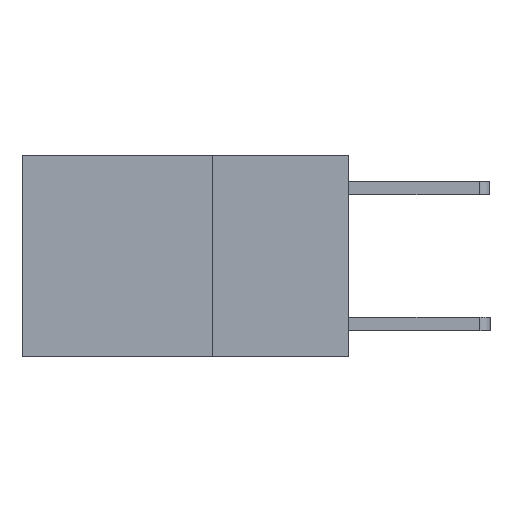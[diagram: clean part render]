
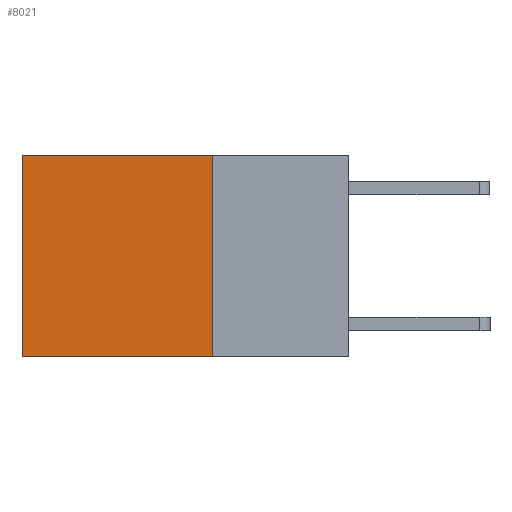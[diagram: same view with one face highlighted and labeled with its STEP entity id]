
A CAD part, left-side view. The second image highlights one B-rep face of the part: STEP entity #8021.
In plain terms, the highlighted planar face has unit normal (-1, 0, 0).
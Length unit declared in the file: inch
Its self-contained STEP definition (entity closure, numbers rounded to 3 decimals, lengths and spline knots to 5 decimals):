
#5 = VECTOR ( 'NONE', #6315, 39.37008 ) ;
#117 = LINE ( 'NONE', #4311, #6963 ) ;
#563 = EDGE_LOOP ( 'NONE', ( #4893, #7709, #1870, #7414 ) ) ;
#976 = CARTESIAN_POINT ( 'NONE',  ( 0.2625, 0.6, 0. ) ) ;
#1108 = LINE ( 'NONE', #2004, #7774 ) ;
#1376 = CARTESIAN_POINT ( 'NONE',  ( 0.2625, 0.25, 0. ) ) ;
#1395 = VECTOR ( 'NONE', #7328, 39.37008 ) ;
#1697 = LINE ( 'NONE', #1863, #5 ) ;
#1863 = CARTESIAN_POINT ( 'NONE',  ( 0.2625, 0.25, -0.37 ) ) ;
#1870 = ORIENTED_EDGE ( 'NONE', *, *, #1940, .F. ) ;
#1940 = EDGE_CURVE ( 'NONE', #6116, #1963, #1108, .T. ) ;
#1963 = VERTEX_POINT ( 'NONE', #6787 ) ;
#2004 = CARTESIAN_POINT ( 'NONE',  ( 0.2625, 0.25, 0. ) ) ;
#2179 = VERTEX_POINT ( 'NONE', #5492 ) ;
#2202 = FACE_OUTER_BOUND ( 'NONE', #563, .T. ) ;
#2701 = PLANE ( 'NONE',  #3496 ) ;
#3143 = EDGE_CURVE ( 'NONE', #6769, #2179, #117, .T. ) ;
#3154 = LINE ( 'NONE', #6671, #1395 ) ;
#3367 = DIRECTION ( 'NONE',  ( 0., 0., -1. ) ) ;
#3496 = AXIS2_PLACEMENT_3D ( 'NONE', #1376, #7406, #3367 ) ;
#3889 = EDGE_CURVE ( 'NONE', #1963, #2179, #1697, .T. ) ;
#4311 = CARTESIAN_POINT ( 'NONE',  ( 0.2625, 0.6, 0. ) ) ;
#4811 = DIRECTION ( 'NONE',  ( 0., 0., -1. ) ) ;
#4893 = ORIENTED_EDGE ( 'NONE', *, *, #3143, .T. ) ;
#4919 = CARTESIAN_POINT ( 'NONE',  ( 0.2625, 0.25, 0. ) ) ;
#5069 = DIRECTION ( 'NONE',  ( 0., 0., -1. ) ) ;
#5492 = CARTESIAN_POINT ( 'NONE',  ( 0.2625, 0.6, -0.37 ) ) ;
#5862 = EDGE_CURVE ( 'NONE', #6116, #6769, #3154, .T. ) ;
#6116 = VERTEX_POINT ( 'NONE', #4919 ) ;
#6315 = DIRECTION ( 'NONE',  ( 0., 1., 0. ) ) ;
#6671 = CARTESIAN_POINT ( 'NONE',  ( 0.2625, 0.25, 0. ) ) ;
#6769 = VERTEX_POINT ( 'NONE', #976 ) ;
#6787 = CARTESIAN_POINT ( 'NONE',  ( 0.2625, 0.25, -0.37 ) ) ;
#6963 = VECTOR ( 'NONE', #5069, 39.37008 ) ;
#7328 = DIRECTION ( 'NONE',  ( 0., 1., 0. ) ) ;
#7406 = DIRECTION ( 'NONE',  ( 1., 0., 0. ) ) ;
#7414 = ORIENTED_EDGE ( 'NONE', *, *, #5862, .T. ) ;
#7709 = ORIENTED_EDGE ( 'NONE', *, *, #3889, .F. ) ;
#7774 = VECTOR ( 'NONE', #4811, 39.37008 ) ;
#8021 = ADVANCED_FACE ( 'NONE', ( #2202 ), #2701, .F. ) ;
